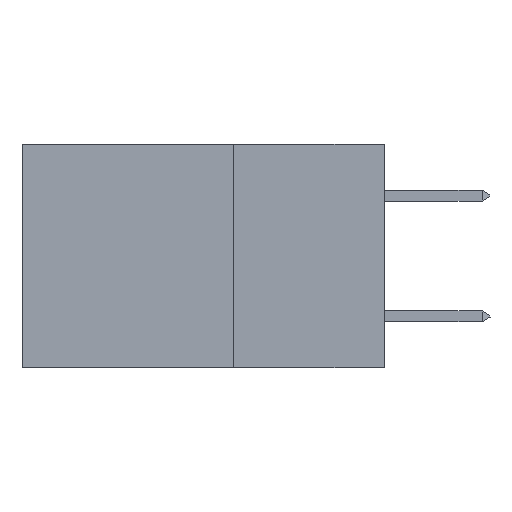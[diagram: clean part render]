
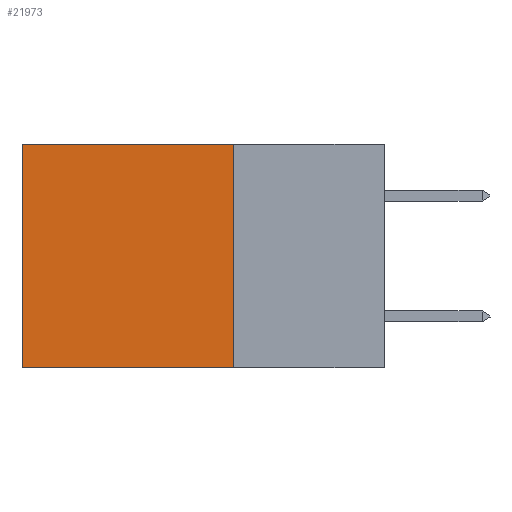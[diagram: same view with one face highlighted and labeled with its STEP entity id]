
A CAD part, left-side view. The second image highlights one B-rep face of the part: STEP entity #21973.
In plain terms, the highlighted planar face has unit normal (-1, 0, 0).
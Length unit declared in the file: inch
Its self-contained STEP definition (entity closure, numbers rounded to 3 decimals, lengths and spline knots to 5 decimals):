
#449 = ORIENTED_EDGE ( 'NONE', *, *, #32154, .T. ) ;
#715 = EDGE_LOOP ( 'NONE', ( #449, #24344, #31817, #13291 ) ) ;
#2086 = VECTOR ( 'NONE', #20671, 39.37008 ) ;
#2180 = VECTOR ( 'NONE', #3983, 39.37008 ) ;
#2439 = VERTEX_POINT ( 'NONE', #27809 ) ;
#3207 = CARTESIAN_POINT ( 'NONE',  ( 0.2875, 0.25, 0. ) ) ;
#3983 = DIRECTION ( 'NONE',  ( 0., 0., -1. ) ) ;
#5846 = VERTEX_POINT ( 'NONE', #30481 ) ;
#5888 = FACE_OUTER_BOUND ( 'NONE', #715, .T. ) ;
#7253 = CARTESIAN_POINT ( 'NONE',  ( 0.2875, 0.6, 0. ) ) ;
#8419 = EDGE_CURVE ( 'NONE', #5846, #32328, #12663, .T. ) ;
#8794 = LINE ( 'NONE', #28329, #2180 ) ;
#10240 = LINE ( 'NONE', #3207, #2086 ) ;
#10365 = CARTESIAN_POINT ( 'NONE',  ( 0.2875, 0.25, -0.37 ) ) ;
#10419 = AXIS2_PLACEMENT_3D ( 'NONE', #14287, #19403, #19298 ) ;
#11823 = VECTOR ( 'NONE', #24708, 39.37008 ) ;
#12663 = LINE ( 'NONE', #10365, #27881 ) ;
#13291 = ORIENTED_EDGE ( 'NONE', *, *, #15603, .T. ) ;
#14287 = CARTESIAN_POINT ( 'NONE',  ( 0.2875, 0.25, 0. ) ) ;
#14335 = EDGE_CURVE ( 'NONE', #2439, #5846, #8794, .T. ) ;
#15150 = CARTESIAN_POINT ( 'NONE',  ( 0.2875, 0.6, -0.37 ) ) ;
#15603 = EDGE_CURVE ( 'NONE', #2439, #17001, #10240, .T. ) ;
#16674 = PLANE ( 'NONE',  #10419 ) ;
#17001 = VERTEX_POINT ( 'NONE', #19644 ) ;
#19298 = DIRECTION ( 'NONE',  ( 0., 0., -1. ) ) ;
#19403 = DIRECTION ( 'NONE',  ( 1., 0., 0. ) ) ;
#19644 = CARTESIAN_POINT ( 'NONE',  ( 0.2875, 0.6, 0. ) ) ;
#20036 = LINE ( 'NONE', #7253, #11823 ) ;
#20671 = DIRECTION ( 'NONE',  ( 0., 1., 0. ) ) ;
#21973 = ADVANCED_FACE ( 'NONE', ( #5888 ), #16674, .F. ) ;
#24344 = ORIENTED_EDGE ( 'NONE', *, *, #8419, .F. ) ;
#24708 = DIRECTION ( 'NONE',  ( 0., 0., -1. ) ) ;
#27809 = CARTESIAN_POINT ( 'NONE',  ( 0.2875, 0.25, 0. ) ) ;
#27881 = VECTOR ( 'NONE', #30186, 39.37008 ) ;
#28329 = CARTESIAN_POINT ( 'NONE',  ( 0.2875, 0.25, 0. ) ) ;
#30186 = DIRECTION ( 'NONE',  ( 0., 1., 0. ) ) ;
#30481 = CARTESIAN_POINT ( 'NONE',  ( 0.2875, 0.25, -0.37 ) ) ;
#31817 = ORIENTED_EDGE ( 'NONE', *, *, #14335, .F. ) ;
#32154 = EDGE_CURVE ( 'NONE', #17001, #32328, #20036, .T. ) ;
#32328 = VERTEX_POINT ( 'NONE', #15150 ) ;
